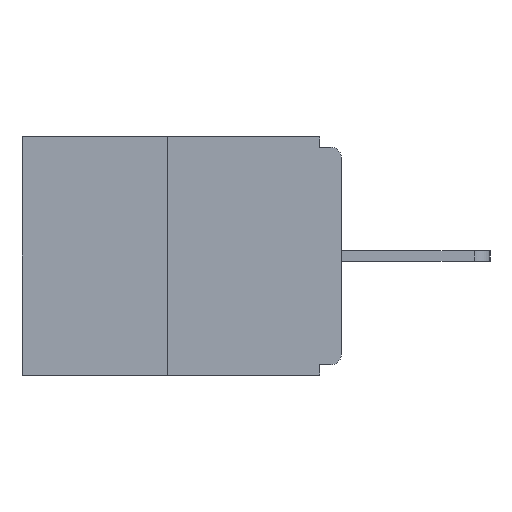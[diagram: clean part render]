
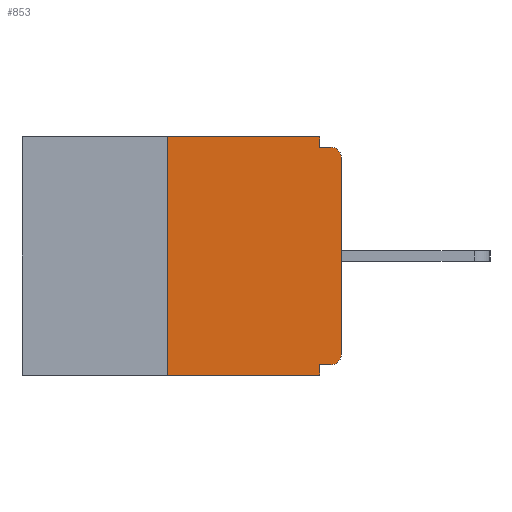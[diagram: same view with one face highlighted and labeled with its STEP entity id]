
A CAD part, left-side view. The second image highlights one B-rep face of the part: STEP entity #853.
In plain terms, the highlighted planar face has unit normal (-1, 0, 0).
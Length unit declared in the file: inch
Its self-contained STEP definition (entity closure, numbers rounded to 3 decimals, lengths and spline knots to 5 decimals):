
#276 = VERTEX_POINT ( 'NONE', #11798 ) ;
#513 = EDGE_CURVE ( 'NONE', #2799, #4512, #6079, .T. ) ;
#515 = LINE ( 'NONE', #16411, #2489 ) ;
#771 = EDGE_CURVE ( 'NONE', #15793, #928, #515, .T. ) ;
#853 = ADVANCED_FACE ( 'NONE', ( #12363 ), #9843, .F. ) ;
#881 = ORIENTED_EDGE ( 'NONE', *, *, #513, .T. ) ;
#928 = VERTEX_POINT ( 'NONE', #7661 ) ;
#1189 = LINE ( 'NONE', #7752, #12758 ) ;
#1364 = CARTESIAN_POINT ( 'NONE',  ( 0., 0.25, 0. ) ) ;
#1995 = DIRECTION ( 'NONE',  ( 0., 0., -1. ) ) ;
#2345 = ORIENTED_EDGE ( 'NONE', *, *, #15077, .T. ) ;
#2489 = VECTOR ( 'NONE', #7001, 39.37008 ) ;
#2735 = AXIS2_PLACEMENT_3D ( 'NONE', #5003, #10118, #15572 ) ;
#2758 = DIRECTION ( 'NONE',  ( 0., 0., -1. ) ) ;
#2799 = VERTEX_POINT ( 'NONE', #15562 ) ;
#2937 = VERTEX_POINT ( 'NONE', #1364 ) ;
#3363 = VECTOR ( 'NONE', #11995, 39.37008 ) ;
#3475 = ORIENTED_EDGE ( 'NONE', *, *, #10178, .T. ) ;
#3497 = DIRECTION ( 'NONE',  ( 0., 0., -1. ) ) ;
#3782 = AXIS2_PLACEMENT_3D ( 'NONE', #8729, #14007, #3497 ) ;
#4512 = VERTEX_POINT ( 'NONE', #15700 ) ;
#4514 = EDGE_CURVE ( 'NONE', #16631, #928, #11551, .T. ) ;
#4686 = AXIS2_PLACEMENT_3D ( 'NONE', #5774, #7163, #15138 ) ;
#4707 = VECTOR ( 'NONE', #2758, 39.37008 ) ;
#4799 = DIRECTION ( 'NONE',  ( 0., 1., 0. ) ) ;
#4885 = CARTESIAN_POINT ( 'NONE',  ( 0., 0.25, -0.343 ) ) ;
#4890 = ORIENTED_EDGE ( 'NONE', *, *, #13958, .F. ) ;
#5003 = CARTESIAN_POINT ( 'NONE',  ( 0., 0.015, -0.313 ) ) ;
#5388 = LINE ( 'NONE', #9547, #3363 ) ;
#5774 = CARTESIAN_POINT ( 'NONE',  ( 0., 0.46, 0. ) ) ;
#5976 = LINE ( 'NONE', #11256, #16583 ) ;
#6079 = CIRCLE ( 'NONE', #2735, 0.015 ) ;
#6521 = CARTESIAN_POINT ( 'NONE',  ( 0., 0.031, -0.343 ) ) ;
#6788 = CARTESIAN_POINT ( 'NONE',  ( 0., 0.031, -0.328 ) ) ;
#7001 = DIRECTION ( 'NONE',  ( 0., -1., 0. ) ) ;
#7163 = DIRECTION ( 'NONE',  ( 1., 0., 0. ) ) ;
#7244 = VECTOR ( 'NONE', #11758, 39.37008 ) ;
#7304 = VERTEX_POINT ( 'NONE', #6521 ) ;
#7661 = CARTESIAN_POINT ( 'NONE',  ( 0., 0.015, -0.015 ) ) ;
#7752 = CARTESIAN_POINT ( 'NONE',  ( 0., 0., -0.328 ) ) ;
#7817 = EDGE_LOOP ( 'NONE', ( #8438, #4890, #2345, #15102, #13471, #881, #3475, #11002, #8181, #14841 ) ) ;
#7961 = CARTESIAN_POINT ( 'NONE',  ( 0., 0.031, -0.343 ) ) ;
#8181 = ORIENTED_EDGE ( 'NONE', *, *, #771, .F. ) ;
#8434 = LINE ( 'NONE', #13698, #7244 ) ;
#8438 = ORIENTED_EDGE ( 'NONE', *, *, #10221, .F. ) ;
#8696 = CARTESIAN_POINT ( 'NONE',  ( 0., 0.031, -0.015 ) ) ;
#8729 = CARTESIAN_POINT ( 'NONE',  ( 0., 0.015, -0.03 ) ) ;
#9465 = VECTOR ( 'NONE', #11034, 39.37008 ) ;
#9547 = CARTESIAN_POINT ( 'NONE',  ( 0., 0., 0. ) ) ;
#9629 = CARTESIAN_POINT ( 'NONE',  ( 0., 0.46, 0. ) ) ;
#9843 = PLANE ( 'NONE',  #4686 ) ;
#10118 = DIRECTION ( 'NONE',  ( -1., 0., 0. ) ) ;
#10178 = EDGE_CURVE ( 'NONE', #4512, #16631, #5388, .T. ) ;
#10221 = EDGE_CURVE ( 'NONE', #2937, #276, #10681, .T. ) ;
#10681 = LINE ( 'NONE', #9629, #15264 ) ;
#11002 = ORIENTED_EDGE ( 'NONE', *, *, #4514, .T. ) ;
#11034 = DIRECTION ( 'NONE',  ( 0., -1., 0. ) ) ;
#11256 = CARTESIAN_POINT ( 'NONE',  ( 0., 0.031, 0. ) ) ;
#11551 = CIRCLE ( 'NONE', #3782, 0.015 ) ;
#11758 = DIRECTION ( 'NONE',  ( 0., 0., 1. ) ) ;
#11798 = CARTESIAN_POINT ( 'NONE',  ( 0., 0.031, 0. ) ) ;
#11995 = DIRECTION ( 'NONE',  ( 0., 0., 1. ) ) ;
#12342 = LINE ( 'NONE', #15035, #9465 ) ;
#12363 = FACE_OUTER_BOUND ( 'NONE', #7817, .T. ) ;
#12689 = VERTEX_POINT ( 'NONE', #6788 ) ;
#12758 = VECTOR ( 'NONE', #4799, 39.37008 ) ;
#13077 = EDGE_CURVE ( 'NONE', #12689, #7304, #15831, .T. ) ;
#13198 = EDGE_CURVE ( 'NONE', #276, #15793, #5976, .T. ) ;
#13471 = ORIENTED_EDGE ( 'NONE', *, *, #13749, .F. ) ;
#13698 = CARTESIAN_POINT ( 'NONE',  ( 0., 0.25, 0. ) ) ;
#13749 = EDGE_CURVE ( 'NONE', #2799, #12689, #1189, .T. ) ;
#13958 = EDGE_CURVE ( 'NONE', #16197, #2937, #8434, .T. ) ;
#14007 = DIRECTION ( 'NONE',  ( -1., 0., 0. ) ) ;
#14263 = CARTESIAN_POINT ( 'NONE',  ( 0., 0., -0.03 ) ) ;
#14841 = ORIENTED_EDGE ( 'NONE', *, *, #13198, .F. ) ;
#15035 = CARTESIAN_POINT ( 'NONE',  ( 0., 0.46, -0.343 ) ) ;
#15077 = EDGE_CURVE ( 'NONE', #16197, #7304, #12342, .T. ) ;
#15102 = ORIENTED_EDGE ( 'NONE', *, *, #13077, .F. ) ;
#15138 = DIRECTION ( 'NONE',  ( 0., 0., -1. ) ) ;
#15264 = VECTOR ( 'NONE', #16273, 39.37008 ) ;
#15562 = CARTESIAN_POINT ( 'NONE',  ( 0., 0.015, -0.328 ) ) ;
#15572 = DIRECTION ( 'NONE',  ( 0., 0., -1. ) ) ;
#15700 = CARTESIAN_POINT ( 'NONE',  ( 0., 0., -0.313 ) ) ;
#15793 = VERTEX_POINT ( 'NONE', #8696 ) ;
#15831 = LINE ( 'NONE', #7961, #4707 ) ;
#16197 = VERTEX_POINT ( 'NONE', #4885 ) ;
#16273 = DIRECTION ( 'NONE',  ( 0., -1., 0. ) ) ;
#16411 = CARTESIAN_POINT ( 'NONE',  ( 0., 0., -0.015 ) ) ;
#16583 = VECTOR ( 'NONE', #1995, 39.37008 ) ;
#16631 = VERTEX_POINT ( 'NONE', #14263 ) ;
